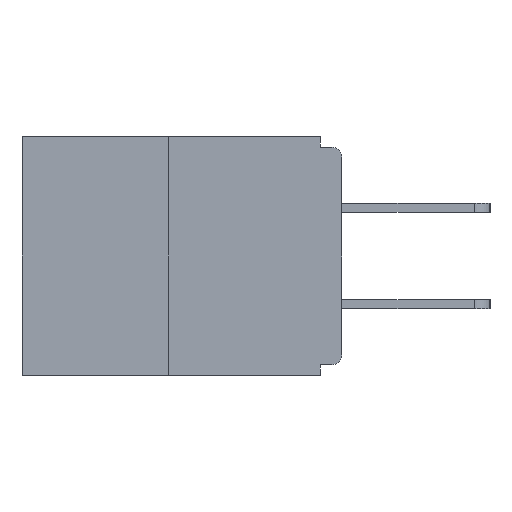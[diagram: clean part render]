
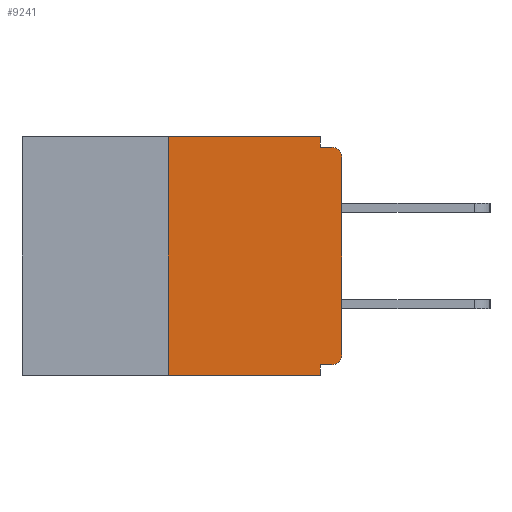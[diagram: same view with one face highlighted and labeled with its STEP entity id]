
A CAD part, left-side view. The second image highlights one B-rep face of the part: STEP entity #9241.
In plain terms, the highlighted planar face has unit normal (-1, 0, 0).
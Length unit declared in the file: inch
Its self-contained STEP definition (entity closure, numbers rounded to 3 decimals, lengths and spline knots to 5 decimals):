
#313 = ORIENTED_EDGE ( 'NONE', *, *, #10445, .T. ) ;
#321 = VECTOR ( 'NONE', #1798, 39.37008 ) ;
#747 = LINE ( 'NONE', #6679, #3955 ) ;
#899 = CARTESIAN_POINT ( 'NONE',  ( 0., 0.25, -0.343 ) ) ;
#942 = DIRECTION ( 'NONE',  ( 1., 0., 0. ) ) ;
#1008 = EDGE_CURVE ( 'NONE', #13396, #7312, #8041, .T. ) ;
#1072 = LINE ( 'NONE', #1628, #5472 ) ;
#1628 = CARTESIAN_POINT ( 'NONE',  ( 0., 0.46, -0.343 ) ) ;
#1798 = DIRECTION ( 'NONE',  ( 0., -1., 0. ) ) ;
#1901 = DIRECTION ( 'NONE',  ( 0., 0., -1. ) ) ;
#2035 = EDGE_CURVE ( 'NONE', #2997, #13396, #3575, .T. ) ;
#2221 = ORIENTED_EDGE ( 'NONE', *, *, #14599, .F. ) ;
#2335 = ORIENTED_EDGE ( 'NONE', *, *, #1008, .F. ) ;
#2895 = VECTOR ( 'NONE', #15675, 39.37008 ) ;
#2997 = VERTEX_POINT ( 'NONE', #9534 ) ;
#3091 = VERTEX_POINT ( 'NONE', #14022 ) ;
#3099 = EDGE_CURVE ( 'NONE', #11226, #11170, #5077, .T. ) ;
#3138 = ORIENTED_EDGE ( 'NONE', *, *, #3099, .F. ) ;
#3247 = ORIENTED_EDGE ( 'NONE', *, *, #2035, .F. ) ;
#3395 = DIRECTION ( 'NONE',  ( 0., 0., -1. ) ) ;
#3575 = LINE ( 'NONE', #13363, #14412 ) ;
#3657 = EDGE_CURVE ( 'NONE', #2997, #10946, #4870, .T. ) ;
#3777 = DIRECTION ( 'NONE',  ( 0., 0., -1. ) ) ;
#3929 = DIRECTION ( 'NONE',  ( -1., 0., 0. ) ) ;
#3955 = VECTOR ( 'NONE', #10402, 39.37008 ) ;
#4294 = EDGE_CURVE ( 'NONE', #11170, #12967, #12622, .T. ) ;
#4509 = ORIENTED_EDGE ( 'NONE', *, *, #3657, .T. ) ;
#4870 = CIRCLE ( 'NONE', #7361, 0.015 ) ;
#4968 = CARTESIAN_POINT ( 'NONE',  ( 0., 0.031, -0.015 ) ) ;
#5048 = CARTESIAN_POINT ( 'NONE',  ( 0., 0.031, 0. ) ) ;
#5077 = LINE ( 'NONE', #11487, #321 ) ;
#5435 = EDGE_CURVE ( 'NONE', #14706, #11226, #10830, .T. ) ;
#5472 = VECTOR ( 'NONE', #13797, 39.37008 ) ;
#5943 = CARTESIAN_POINT ( 'NONE',  ( 0., 0.031, -0.343 ) ) ;
#6340 = DIRECTION ( 'NONE',  ( 0., 0., -1. ) ) ;
#6397 = ORIENTED_EDGE ( 'NONE', *, *, #9755, .T. ) ;
#6679 = CARTESIAN_POINT ( 'NONE',  ( 0., 0., -0.015 ) ) ;
#6770 = ORIENTED_EDGE ( 'NONE', *, *, #4294, .F. ) ;
#6926 = VERTEX_POINT ( 'NONE', #7376 ) ;
#7029 = CIRCLE ( 'NONE', #7837, 0.015 ) ;
#7043 = CARTESIAN_POINT ( 'NONE',  ( 0., 0.46, 0. ) ) ;
#7312 = VERTEX_POINT ( 'NONE', #15690 ) ;
#7361 = AXIS2_PLACEMENT_3D ( 'NONE', #7609, #3929, #3777 ) ;
#7376 = CARTESIAN_POINT ( 'NONE',  ( 0., 0.015, -0.015 ) ) ;
#7609 = CARTESIAN_POINT ( 'NONE',  ( 0., 0.015, -0.313 ) ) ;
#7837 = AXIS2_PLACEMENT_3D ( 'NONE', #13883, #10780, #1901 ) ;
#8041 = LINE ( 'NONE', #5943, #15246 ) ;
#8378 = DIRECTION ( 'NONE',  ( 0., 0., 1. ) ) ;
#8867 = CARTESIAN_POINT ( 'NONE',  ( 0., 0.25, 0. ) ) ;
#8926 = CARTESIAN_POINT ( 'NONE',  ( 0., 0.031, 0. ) ) ;
#9186 = EDGE_LOOP ( 'NONE', ( #3138, #14336, #313, #2335, #3247, #4509, #13107, #6397, #2221, #6770 ) ) ;
#9241 = ADVANCED_FACE ( 'NONE', ( #11360 ), #10763, .F. ) ;
#9242 = CARTESIAN_POINT ( 'NONE',  ( 0., 0., 0. ) ) ;
#9534 = CARTESIAN_POINT ( 'NONE',  ( 0., 0.015, -0.328 ) ) ;
#9606 = CARTESIAN_POINT ( 'NONE',  ( 0., 0.25, 0. ) ) ;
#9755 = EDGE_CURVE ( 'NONE', #3091, #6926, #7029, .T. ) ;
#10402 = DIRECTION ( 'NONE',  ( 0., -1., 0. ) ) ;
#10445 = EDGE_CURVE ( 'NONE', #14706, #7312, #1072, .T. ) ;
#10677 = EDGE_CURVE ( 'NONE', #10946, #3091, #12850, .T. ) ;
#10763 = PLANE ( 'NONE',  #12719 ) ;
#10780 = DIRECTION ( 'NONE',  ( -1., 0., 0. ) ) ;
#10810 = DIRECTION ( 'NONE',  ( 0., 0., -1. ) ) ;
#10830 = LINE ( 'NONE', #9606, #2895 ) ;
#10946 = VERTEX_POINT ( 'NONE', #11095 ) ;
#11073 = VECTOR ( 'NONE', #6340, 39.37008 ) ;
#11095 = CARTESIAN_POINT ( 'NONE',  ( 0., 0., -0.313 ) ) ;
#11115 = VECTOR ( 'NONE', #8378, 39.37008 ) ;
#11170 = VERTEX_POINT ( 'NONE', #8926 ) ;
#11226 = VERTEX_POINT ( 'NONE', #8867 ) ;
#11360 = FACE_OUTER_BOUND ( 'NONE', #9186, .T. ) ;
#11487 = CARTESIAN_POINT ( 'NONE',  ( 0., 0.46, 0. ) ) ;
#11957 = DIRECTION ( 'NONE',  ( 0., 1., 0. ) ) ;
#12622 = LINE ( 'NONE', #5048, #11073 ) ;
#12719 = AXIS2_PLACEMENT_3D ( 'NONE', #7043, #942, #10810 ) ;
#12850 = LINE ( 'NONE', #9242, #11115 ) ;
#12967 = VERTEX_POINT ( 'NONE', #4968 ) ;
#13107 = ORIENTED_EDGE ( 'NONE', *, *, #10677, .T. ) ;
#13363 = CARTESIAN_POINT ( 'NONE',  ( 0., 0., -0.328 ) ) ;
#13396 = VERTEX_POINT ( 'NONE', #14034 ) ;
#13797 = DIRECTION ( 'NONE',  ( 0., -1., 0. ) ) ;
#13883 = CARTESIAN_POINT ( 'NONE',  ( 0., 0.015, -0.03 ) ) ;
#14022 = CARTESIAN_POINT ( 'NONE',  ( 0., 0., -0.03 ) ) ;
#14034 = CARTESIAN_POINT ( 'NONE',  ( 0., 0.031, -0.328 ) ) ;
#14336 = ORIENTED_EDGE ( 'NONE', *, *, #5435, .F. ) ;
#14412 = VECTOR ( 'NONE', #11957, 39.37008 ) ;
#14599 = EDGE_CURVE ( 'NONE', #12967, #6926, #747, .T. ) ;
#14706 = VERTEX_POINT ( 'NONE', #899 ) ;
#15246 = VECTOR ( 'NONE', #3395, 39.37008 ) ;
#15675 = DIRECTION ( 'NONE',  ( 0., 0., 1. ) ) ;
#15690 = CARTESIAN_POINT ( 'NONE',  ( 0., 0.031, -0.343 ) ) ;
